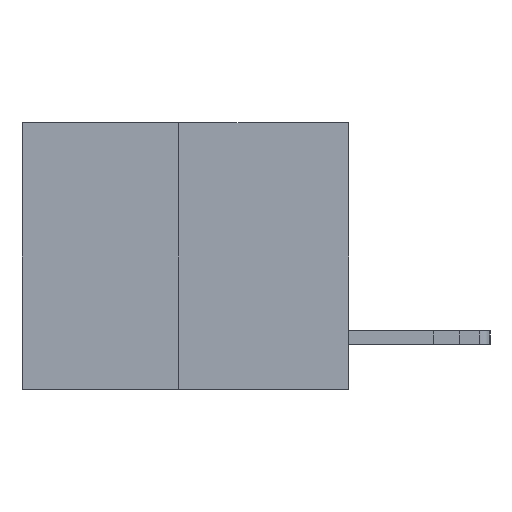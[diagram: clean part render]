
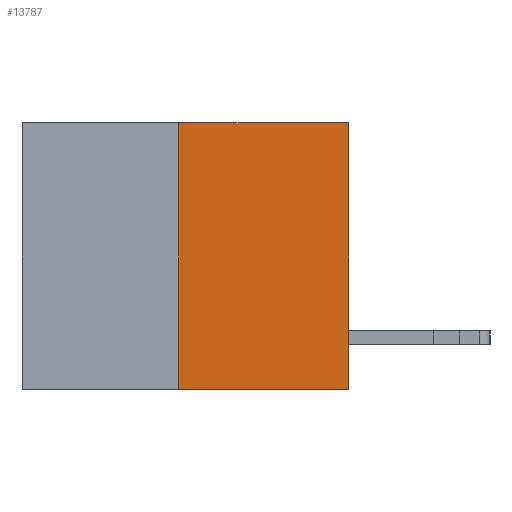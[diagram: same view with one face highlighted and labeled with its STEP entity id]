
A CAD part, left-side view. The second image highlights one B-rep face of the part: STEP entity #13787.
In plain terms, the highlighted planar face has unit normal (-1, 0, 0).
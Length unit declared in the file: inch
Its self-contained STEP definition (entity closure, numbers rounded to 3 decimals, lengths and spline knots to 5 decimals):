
#396 = LINE ( 'NONE', #11664, #5808 ) ;
#708 = EDGE_CURVE ( 'NONE', #5235, #7091, #5160, .T. ) ;
#1048 = DIRECTION ( 'NONE',  ( 0., 0., -1. ) ) ;
#1157 = LINE ( 'NONE', #11861, #14425 ) ;
#1592 = DIRECTION ( 'NONE',  ( 0., -1., 0. ) ) ;
#1871 = CARTESIAN_POINT ( 'NONE',  ( 0., 0., 0. ) ) ;
#1897 = LINE ( 'NONE', #16453, #4706 ) ;
#1938 = EDGE_CURVE ( 'NONE', #5604, #3218, #396, .T. ) ;
#1941 = CARTESIAN_POINT ( 'NONE',  ( 0., 0.312, 0. ) ) ;
#3218 = VERTEX_POINT ( 'NONE', #1871 ) ;
#4052 = DIRECTION ( 'NONE',  ( 0., -1., 0. ) ) ;
#4159 = EDGE_LOOP ( 'NONE', ( #4630, #14421, #6066, #10523 ) ) ;
#4630 = ORIENTED_EDGE ( 'NONE', *, *, #13485, .F. ) ;
#4706 = VECTOR ( 'NONE', #8746, 39.37008 ) ;
#5160 = LINE ( 'NONE', #13280, #10189 ) ;
#5235 = VERTEX_POINT ( 'NONE', #10114 ) ;
#5604 = VERTEX_POINT ( 'NONE', #1941 ) ;
#5808 = VECTOR ( 'NONE', #4052, 39.37008 ) ;
#6066 = ORIENTED_EDGE ( 'NONE', *, *, #6499, .T. ) ;
#6132 = PLANE ( 'NONE',  #12723 ) ;
#6499 = EDGE_CURVE ( 'NONE', #7091, #3218, #1157, .T. ) ;
#7091 = VERTEX_POINT ( 'NONE', #10615 ) ;
#7122 = FACE_OUTER_BOUND ( 'NONE', #4159, .T. ) ;
#8746 = DIRECTION ( 'NONE',  ( 0., 0., 1. ) ) ;
#10104 = DIRECTION ( 'NONE',  ( 0., 0., 1. ) ) ;
#10114 = CARTESIAN_POINT ( 'NONE',  ( 0., 0.312, -0.49 ) ) ;
#10189 = VECTOR ( 'NONE', #1592, 39.37008 ) ;
#10523 = ORIENTED_EDGE ( 'NONE', *, *, #1938, .F. ) ;
#10615 = CARTESIAN_POINT ( 'NONE',  ( 0., 0., -0.49 ) ) ;
#11664 = CARTESIAN_POINT ( 'NONE',  ( 0., 0.6, 0. ) ) ;
#11861 = CARTESIAN_POINT ( 'NONE',  ( 0., 0., 0. ) ) ;
#12723 = AXIS2_PLACEMENT_3D ( 'NONE', #15148, #16451, #1048 ) ;
#13280 = CARTESIAN_POINT ( 'NONE',  ( 0., 0.6, -0.49 ) ) ;
#13485 = EDGE_CURVE ( 'NONE', #5235, #5604, #1897, .T. ) ;
#13787 = ADVANCED_FACE ( 'NONE', ( #7122 ), #6132, .F. ) ;
#14421 = ORIENTED_EDGE ( 'NONE', *, *, #708, .T. ) ;
#14425 = VECTOR ( 'NONE', #10104, 39.37008 ) ;
#15148 = CARTESIAN_POINT ( 'NONE',  ( 0., 0.6, 0. ) ) ;
#16451 = DIRECTION ( 'NONE',  ( 1., 0., 0. ) ) ;
#16453 = CARTESIAN_POINT ( 'NONE',  ( 0., 0.312, -0.49 ) ) ;
